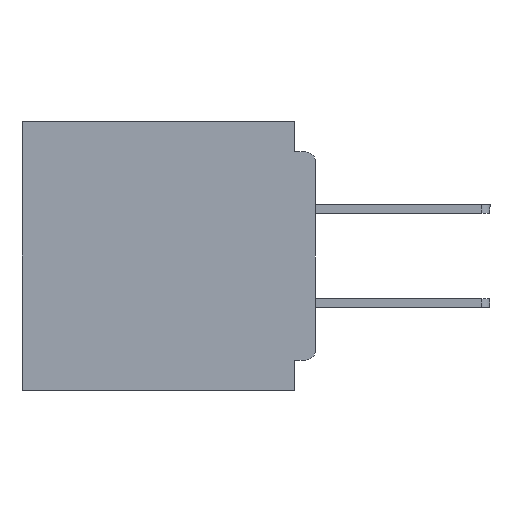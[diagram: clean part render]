
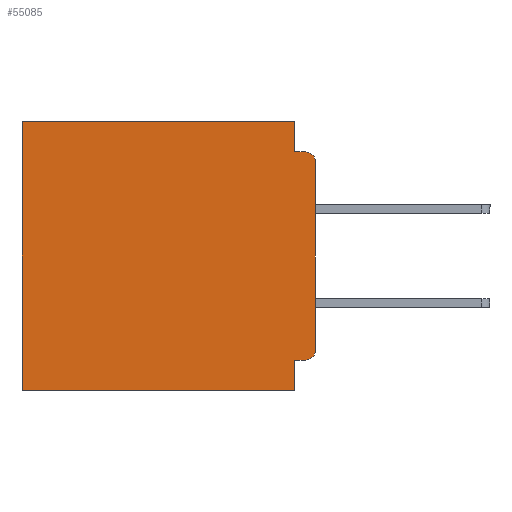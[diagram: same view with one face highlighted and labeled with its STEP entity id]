
A CAD part, left-side view. The second image highlights one B-rep face of the part: STEP entity #55085.
In plain terms, the highlighted planar face has unit normal (-1, 0, 0).
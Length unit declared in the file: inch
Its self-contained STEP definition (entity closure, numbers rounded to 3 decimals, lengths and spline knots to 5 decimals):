
#77 = VECTOR ( 'NONE', #9879, 39.37008 ) ;
#142 = EDGE_CURVE ( 'NONE', #41205, #11666, #28897, .T. ) ;
#516 = DIRECTION ( 'NONE',  ( 0., 1., 0. ) ) ;
#546 = DIRECTION ( 'NONE',  ( 0., 0., -1. ) ) ;
#1980 = VERTEX_POINT ( 'NONE', #26110 ) ;
#2869 = CIRCLE ( 'NONE', #35642, 0.015 ) ;
#3335 = LINE ( 'NONE', #51370, #47978 ) ;
#3894 = VECTOR ( 'NONE', #31745, 39.37008 ) ;
#6742 = EDGE_CURVE ( 'NONE', #25952, #26821, #52554, .T. ) ;
#6839 = EDGE_CURVE ( 'NONE', #15490, #55763, #48531, .T. ) ;
#7033 = CARTESIAN_POINT ( 'NONE',  ( 0.3, 0.031, -0.4 ) ) ;
#7081 = EDGE_CURVE ( 'NONE', #55763, #26821, #47839, .T. ) ;
#7966 = ORIENTED_EDGE ( 'NONE', *, *, #37710, .F. ) ;
#8275 = DIRECTION ( 'NONE',  ( 0., 0., -1. ) ) ;
#9879 = DIRECTION ( 'NONE',  ( 0., 0., -1. ) ) ;
#10302 = CARTESIAN_POINT ( 'NONE',  ( 0.3, 0., -0.4 ) ) ;
#11083 = CARTESIAN_POINT ( 'NONE',  ( 0.3, 0., -0.355 ) ) ;
#11666 = VERTEX_POINT ( 'NONE', #34517 ) ;
#11808 = ORIENTED_EDGE ( 'NONE', *, *, #7081, .T. ) ;
#11845 = VECTOR ( 'NONE', #46371, 39.37008 ) ;
#12024 = CARTESIAN_POINT ( 'NONE',  ( 0.3, 0.015, -0.06 ) ) ;
#13228 = VERTEX_POINT ( 'NONE', #19697 ) ;
#13440 = LINE ( 'NONE', #45409, #46566 ) ;
#14694 = DIRECTION ( 'NONE',  ( 0., 0., -1. ) ) ;
#15490 = VERTEX_POINT ( 'NONE', #27034 ) ;
#16298 = FACE_OUTER_BOUND ( 'NONE', #33264, .T. ) ;
#16404 = DIRECTION ( 'NONE',  ( 0., 0., -1. ) ) ;
#16478 = ORIENTED_EDGE ( 'NONE', *, *, #29634, .F. ) ;
#17378 = VECTOR ( 'NONE', #516, 39.37008 ) ;
#18223 = CARTESIAN_POINT ( 'NONE',  ( 0.3, 0.031, -0.4 ) ) ;
#18384 = DIRECTION ( 'NONE',  ( 0., 1., 0. ) ) ;
#19697 = CARTESIAN_POINT ( 'NONE',  ( 0.3, 0., -0.06 ) ) ;
#20115 = AXIS2_PLACEMENT_3D ( 'NONE', #52304, #26515, #546 ) ;
#20621 = CARTESIAN_POINT ( 'NONE',  ( 0.3, 0., -0.34 ) ) ;
#22778 = ORIENTED_EDGE ( 'NONE', *, *, #6742, .F. ) ;
#23213 = PLANE ( 'NONE',  #42722 ) ;
#24539 = LINE ( 'NONE', #18223, #77 ) ;
#24814 = CARTESIAN_POINT ( 'NONE',  ( 0.3, 0.437, -0.4 ) ) ;
#24925 = VECTOR ( 'NONE', #46295, 39.37008 ) ;
#25952 = VERTEX_POINT ( 'NONE', #7033 ) ;
#26110 = CARTESIAN_POINT ( 'NONE',  ( 0.3, 0.031, -0.045 ) ) ;
#26515 = DIRECTION ( 'NONE',  ( -1., 0., 0. ) ) ;
#26821 = VERTEX_POINT ( 'NONE', #29852 ) ;
#27034 = CARTESIAN_POINT ( 'NONE',  ( 0.3, 0.031, 0. ) ) ;
#28050 = ORIENTED_EDGE ( 'NONE', *, *, #31367, .F. ) ;
#28222 = CARTESIAN_POINT ( 'NONE',  ( 0.3, 0.437, 0. ) ) ;
#28897 = LINE ( 'NONE', #11083, #17378 ) ;
#29634 = EDGE_CURVE ( 'NONE', #13228, #51809, #37542, .T. ) ;
#29852 = CARTESIAN_POINT ( 'NONE',  ( 0.3, 0.437, -0.4 ) ) ;
#30136 = VERTEX_POINT ( 'NONE', #45592 ) ;
#30925 = EDGE_CURVE ( 'NONE', #13228, #30136, #2869, .T. ) ;
#31367 = EDGE_CURVE ( 'NONE', #11666, #25952, #24539, .T. ) ;
#31745 = DIRECTION ( 'NONE',  ( 0., 1., 0. ) ) ;
#32071 = ORIENTED_EDGE ( 'NONE', *, *, #30925, .T. ) ;
#33264 = EDGE_LOOP ( 'NONE', ( #16478, #32071, #39624, #7966, #38938, #11808, #22778, #28050, #38283, #37517 ) ) ;
#34517 = CARTESIAN_POINT ( 'NONE',  ( 0.3, 0.031, -0.355 ) ) ;
#35642 = AXIS2_PLACEMENT_3D ( 'NONE', #12024, #42297, #16404 ) ;
#36110 = CARTESIAN_POINT ( 'NONE',  ( 0.3, 0., 0. ) ) ;
#37517 = ORIENTED_EDGE ( 'NONE', *, *, #51429, .T. ) ;
#37542 = LINE ( 'NONE', #42059, #11845 ) ;
#37710 = EDGE_CURVE ( 'NONE', #15490, #1980, #3335, .T. ) ;
#38283 = ORIENTED_EDGE ( 'NONE', *, *, #142, .F. ) ;
#38938 = ORIENTED_EDGE ( 'NONE', *, *, #6839, .T. ) ;
#39624 = ORIENTED_EDGE ( 'NONE', *, *, #42990, .F. ) ;
#39900 = CARTESIAN_POINT ( 'NONE',  ( 0.3, 0., -0.4 ) ) ;
#40576 = DIRECTION ( 'NONE',  ( 1., 0., 0. ) ) ;
#41059 = DIRECTION ( 'NONE',  ( 0., -1., 0. ) ) ;
#41205 = VERTEX_POINT ( 'NONE', #44642 ) ;
#42059 = CARTESIAN_POINT ( 'NONE',  ( 0.3, 0., -0.4 ) ) ;
#42297 = DIRECTION ( 'NONE',  ( -1., 0., 0. ) ) ;
#42722 = AXIS2_PLACEMENT_3D ( 'NONE', #10302, #40576, #14694 ) ;
#42990 = EDGE_CURVE ( 'NONE', #1980, #30136, #13440, .T. ) ;
#44642 = CARTESIAN_POINT ( 'NONE',  ( 0.3, 0.015, -0.355 ) ) ;
#45003 = CIRCLE ( 'NONE', #20115, 0.015 ) ;
#45409 = CARTESIAN_POINT ( 'NONE',  ( 0.3, 0., -0.045 ) ) ;
#45592 = CARTESIAN_POINT ( 'NONE',  ( 0.3, 0.015, -0.045 ) ) ;
#46295 = DIRECTION ( 'NONE',  ( 0., 0., -1. ) ) ;
#46371 = DIRECTION ( 'NONE',  ( 0., 0., -1. ) ) ;
#46566 = VECTOR ( 'NONE', #41059, 39.37008 ) ;
#47839 = LINE ( 'NONE', #24814, #24925 ) ;
#47978 = VECTOR ( 'NONE', #8275, 39.37008 ) ;
#48531 = LINE ( 'NONE', #36110, #3894 ) ;
#51240 = VECTOR ( 'NONE', #18384, 39.37008 ) ;
#51370 = CARTESIAN_POINT ( 'NONE',  ( 0.3, 0.031, 0. ) ) ;
#51429 = EDGE_CURVE ( 'NONE', #41205, #51809, #45003, .T. ) ;
#51809 = VERTEX_POINT ( 'NONE', #20621 ) ;
#52304 = CARTESIAN_POINT ( 'NONE',  ( 0.3, 0.015, -0.34 ) ) ;
#52554 = LINE ( 'NONE', #39900, #51240 ) ;
#55085 = ADVANCED_FACE ( 'NONE', ( #16298 ), #23213, .F. ) ;
#55763 = VERTEX_POINT ( 'NONE', #28222 ) ;
